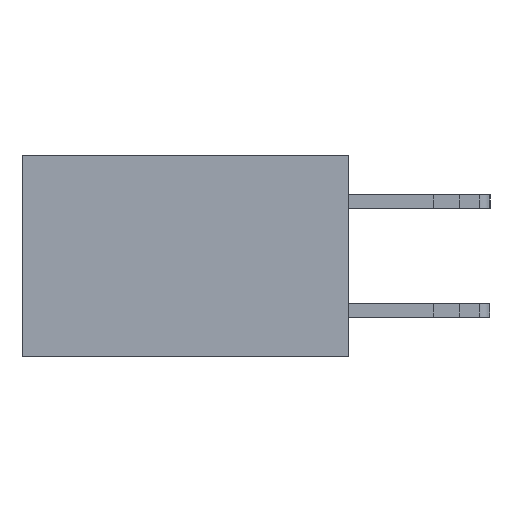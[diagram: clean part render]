
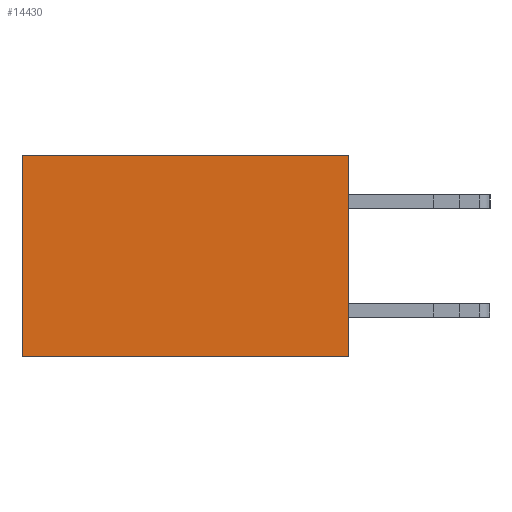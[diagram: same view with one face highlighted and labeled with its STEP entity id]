
A CAD part, left-side view. The second image highlights one B-rep face of the part: STEP entity #14430.
In plain terms, the highlighted planar face has unit normal (-1, 0, 0).
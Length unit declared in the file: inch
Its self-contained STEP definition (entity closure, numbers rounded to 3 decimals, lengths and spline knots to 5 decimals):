
#430 = DIRECTION ( 'NONE',  ( 0., 0., -1. ) ) ;
#660 = DIRECTION ( 'NONE',  ( 0., 0., -1. ) ) ;
#773 = ORIENTED_EDGE ( 'NONE', *, *, #9555, .F. ) ;
#1034 = CARTESIAN_POINT ( 'NONE',  ( 0.298, 0.6, 0. ) ) ;
#1675 = EDGE_CURVE ( 'NONE', #4784, #10560, #3590, .T. ) ;
#1969 = DIRECTION ( 'NONE',  ( 0., 1., 0. ) ) ;
#3590 = LINE ( 'NONE', #14088, #12372 ) ;
#3687 = CARTESIAN_POINT ( 'NONE',  ( 0.298, 0., 0. ) ) ;
#4024 = EDGE_LOOP ( 'NONE', ( #11406, #773, #10781, #5092 ) ) ;
#4771 = PLANE ( 'NONE',  #10689 ) ;
#4784 = VERTEX_POINT ( 'NONE', #3687 ) ;
#5092 = ORIENTED_EDGE ( 'NONE', *, *, #1675, .T. ) ;
#5343 = EDGE_CURVE ( 'NONE', #10560, #12417, #12779, .T. ) ;
#5948 = DIRECTION ( 'NONE',  ( 0., 0., -1. ) ) ;
#6678 = VECTOR ( 'NONE', #660, 39.37008 ) ;
#8237 = CARTESIAN_POINT ( 'NONE',  ( 0.298, 0., -0.37 ) ) ;
#8477 = CARTESIAN_POINT ( 'NONE',  ( 0.298, 0., 0. ) ) ;
#8839 = VERTEX_POINT ( 'NONE', #13539 ) ;
#9426 = LINE ( 'NONE', #8237, #12468 ) ;
#9555 = EDGE_CURVE ( 'NONE', #8839, #12417, #9426, .T. ) ;
#9686 = EDGE_CURVE ( 'NONE', #4784, #8839, #10343, .T. ) ;
#10343 = LINE ( 'NONE', #8477, #12986 ) ;
#10524 = CARTESIAN_POINT ( 'NONE',  ( 0.298, 0., 0. ) ) ;
#10560 = VERTEX_POINT ( 'NONE', #1034 ) ;
#10689 = AXIS2_PLACEMENT_3D ( 'NONE', #10524, #12788, #5948 ) ;
#10781 = ORIENTED_EDGE ( 'NONE', *, *, #9686, .F. ) ;
#10944 = FACE_OUTER_BOUND ( 'NONE', #4024, .T. ) ;
#11406 = ORIENTED_EDGE ( 'NONE', *, *, #5343, .T. ) ;
#12372 = VECTOR ( 'NONE', #1969, 39.37008 ) ;
#12417 = VERTEX_POINT ( 'NONE', #13461 ) ;
#12468 = VECTOR ( 'NONE', #13938, 39.37008 ) ;
#12779 = LINE ( 'NONE', #14389, #6678 ) ;
#12788 = DIRECTION ( 'NONE',  ( 1., 0., 0. ) ) ;
#12986 = VECTOR ( 'NONE', #430, 39.37008 ) ;
#13461 = CARTESIAN_POINT ( 'NONE',  ( 0.298, 0.6, -0.37 ) ) ;
#13539 = CARTESIAN_POINT ( 'NONE',  ( 0.298, 0., -0.37 ) ) ;
#13938 = DIRECTION ( 'NONE',  ( 0., 1., 0. ) ) ;
#14088 = CARTESIAN_POINT ( 'NONE',  ( 0.298, 0., 0. ) ) ;
#14389 = CARTESIAN_POINT ( 'NONE',  ( 0.298, 0.6, 0. ) ) ;
#14430 = ADVANCED_FACE ( 'NONE', ( #10944 ), #4771, .F. ) ;
